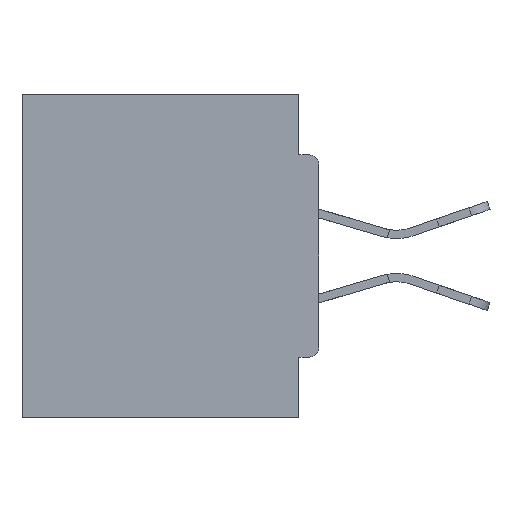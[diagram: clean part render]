
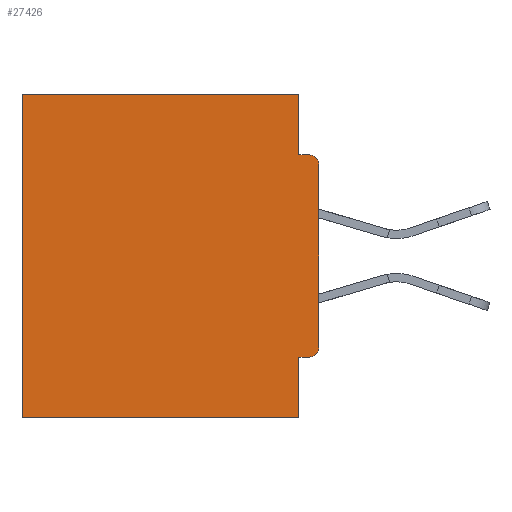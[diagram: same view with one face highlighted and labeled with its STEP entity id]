
A CAD part, left-side view. The second image highlights one B-rep face of the part: STEP entity #27426.
In plain terms, the highlighted planar face has unit normal (-1, 0, 0).
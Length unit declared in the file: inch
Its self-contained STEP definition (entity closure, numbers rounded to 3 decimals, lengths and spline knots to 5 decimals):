
#908 = DIRECTION ( 'NONE',  ( 0., -1., 0. ) ) ;
#1036 = EDGE_CURVE ( 'NONE', #26128, #29385, #31450, .T. ) ;
#2875 = VERTEX_POINT ( 'NONE', #4500 ) ;
#3977 = CARTESIAN_POINT ( 'NONE',  ( 0.298, 0., -0.0935 ) ) ;
#4500 = CARTESIAN_POINT ( 'NONE',  ( 0.298, 0.031, 0. ) ) ;
#4774 = LINE ( 'NONE', #9649, #39396 ) ;
#5343 = EDGE_CURVE ( 'NONE', #30835, #35171, #8415, .T. ) ;
#6039 = AXIS2_PLACEMENT_3D ( 'NONE', #40846, #12125, #31103 ) ;
#6791 = CARTESIAN_POINT ( 'NONE',  ( 0.298, 0.015, -0.3915 ) ) ;
#7238 = CARTESIAN_POINT ( 'NONE',  ( 0.298, 0.015, -0.0935 ) ) ;
#7319 = CARTESIAN_POINT ( 'NONE',  ( 0.298, 0.46, 0. ) ) ;
#7606 = ORIENTED_EDGE ( 'NONE', *, *, #35870, .T. ) ;
#7838 = DIRECTION ( 'NONE',  ( 0., 0., -1. ) ) ;
#8415 = LINE ( 'NONE', #36304, #37063 ) ;
#9649 = CARTESIAN_POINT ( 'NONE',  ( 0.298, 0.031, -0.5 ) ) ;
#10149 = CARTESIAN_POINT ( 'NONE',  ( 0.298, 0.015, -0.1085 ) ) ;
#10353 = DIRECTION ( 'NONE',  ( 0., 0., -1. ) ) ;
#11245 = ORIENTED_EDGE ( 'NONE', *, *, #20241, .T. ) ;
#11386 = ORIENTED_EDGE ( 'NONE', *, *, #24645, .F. ) ;
#12125 = DIRECTION ( 'NONE',  ( 1., 0., 0. ) ) ;
#12894 = EDGE_CURVE ( 'NONE', #2875, #20817, #28044, .T. ) ;
#13307 = ORIENTED_EDGE ( 'NONE', *, *, #5343, .F. ) ;
#14392 = CARTESIAN_POINT ( 'NONE',  ( 0.298, 0., 0. ) ) ;
#14441 = CARTESIAN_POINT ( 'NONE',  ( 0.298, 0.46, 0. ) ) ;
#14449 = VECTOR ( 'NONE', #39808, 39.37008 ) ;
#14754 = ORIENTED_EDGE ( 'NONE', *, *, #37496, .F. ) ;
#14957 = VERTEX_POINT ( 'NONE', #29770 ) ;
#15213 = EDGE_LOOP ( 'NONE', ( #7606, #28467, #11386, #28858, #11245, #13307, #23914, #29874, #31827, #14754 ) ) ;
#16209 = DIRECTION ( 'NONE',  ( -1., 0., 0. ) ) ;
#16326 = CARTESIAN_POINT ( 'NONE',  ( 0.298, 0.031, -0.5 ) ) ;
#20241 = EDGE_CURVE ( 'NONE', #20817, #35171, #28998, .T. ) ;
#20654 = DIRECTION ( 'NONE',  ( 0., 0., -1. ) ) ;
#20817 = VERTEX_POINT ( 'NONE', #7319 ) ;
#21018 = CARTESIAN_POINT ( 'NONE',  ( 0.298, 0., 0. ) ) ;
#21055 = VECTOR ( 'NONE', #908, 39.37008 ) ;
#21296 = DIRECTION ( 'NONE',  ( 0., 1., 0. ) ) ;
#22130 = AXIS2_PLACEMENT_3D ( 'NONE', #6791, #22304, #38011 ) ;
#22304 = DIRECTION ( 'NONE',  ( -1., 0., 0. ) ) ;
#22726 = CIRCLE ( 'NONE', #31453, 0.015 ) ;
#23914 = ORIENTED_EDGE ( 'NONE', *, *, #25435, .F. ) ;
#23992 = CARTESIAN_POINT ( 'NONE',  ( 0.298, 0.46, -0.5 ) ) ;
#24191 = CARTESIAN_POINT ( 'NONE',  ( 0.298, 0.031, -0.0935 ) ) ;
#24201 = VECTOR ( 'NONE', #10353, 39.37008 ) ;
#24645 = EDGE_CURVE ( 'NONE', #2875, #26128, #33553, .T. ) ;
#25435 = EDGE_CURVE ( 'NONE', #28665, #30835, #4774, .T. ) ;
#26027 = FACE_OUTER_BOUND ( 'NONE', #15213, .T. ) ;
#26128 = VERTEX_POINT ( 'NONE', #24191 ) ;
#27426 = ADVANCED_FACE ( 'NONE', ( #26027 ), #34250, .F. ) ;
#28044 = LINE ( 'NONE', #21018, #35411 ) ;
#28341 = LINE ( 'NONE', #30626, #14449 ) ;
#28467 = ORIENTED_EDGE ( 'NONE', *, *, #1036, .F. ) ;
#28665 = VERTEX_POINT ( 'NONE', #29125 ) ;
#28858 = ORIENTED_EDGE ( 'NONE', *, *, #12894, .T. ) ;
#28923 = DIRECTION ( 'NONE',  ( 0., 0., -1. ) ) ;
#28998 = LINE ( 'NONE', #14441, #36326 ) ;
#29125 = CARTESIAN_POINT ( 'NONE',  ( 0.298, 0.031, -0.4065 ) ) ;
#29385 = VERTEX_POINT ( 'NONE', #7238 ) ;
#29770 = CARTESIAN_POINT ( 'NONE',  ( 0.298, 0., -0.3915 ) ) ;
#29874 = ORIENTED_EDGE ( 'NONE', *, *, #38999, .F. ) ;
#30626 = CARTESIAN_POINT ( 'NONE',  ( 0.298, 0., -0.4065 ) ) ;
#30759 = CARTESIAN_POINT ( 'NONE',  ( 0.298, 0., -0.1085 ) ) ;
#30835 = VERTEX_POINT ( 'NONE', #16326 ) ;
#30977 = VECTOR ( 'NONE', #20654, 39.37008 ) ;
#31103 = DIRECTION ( 'NONE',  ( 0., 0., -1. ) ) ;
#31450 = LINE ( 'NONE', #3977, #21055 ) ;
#31453 = AXIS2_PLACEMENT_3D ( 'NONE', #10149, #16209, #35459 ) ;
#31827 = ORIENTED_EDGE ( 'NONE', *, *, #32901, .T. ) ;
#32092 = VERTEX_POINT ( 'NONE', #38429 ) ;
#32901 = EDGE_CURVE ( 'NONE', #32092, #14957, #36401, .T. ) ;
#32926 = LINE ( 'NONE', #14392, #30977 ) ;
#33553 = LINE ( 'NONE', #35662, #24201 ) ;
#34250 = PLANE ( 'NONE',  #6039 ) ;
#34569 = VERTEX_POINT ( 'NONE', #30759 ) ;
#35171 = VERTEX_POINT ( 'NONE', #23992 ) ;
#35411 = VECTOR ( 'NONE', #21296, 39.37008 ) ;
#35459 = DIRECTION ( 'NONE',  ( 0., 0., -1. ) ) ;
#35662 = CARTESIAN_POINT ( 'NONE',  ( 0.298, 0.031, -0.5 ) ) ;
#35870 = EDGE_CURVE ( 'NONE', #34569, #29385, #22726, .T. ) ;
#36180 = DIRECTION ( 'NONE',  ( 0., 1., 0. ) ) ;
#36304 = CARTESIAN_POINT ( 'NONE',  ( 0.298, 0., -0.5 ) ) ;
#36326 = VECTOR ( 'NONE', #7838, 39.37008 ) ;
#36401 = CIRCLE ( 'NONE', #22130, 0.015 ) ;
#37063 = VECTOR ( 'NONE', #36180, 39.37008 ) ;
#37496 = EDGE_CURVE ( 'NONE', #34569, #14957, #32926, .T. ) ;
#38011 = DIRECTION ( 'NONE',  ( 0., 0., -1. ) ) ;
#38429 = CARTESIAN_POINT ( 'NONE',  ( 0.298, 0.015, -0.4065 ) ) ;
#38999 = EDGE_CURVE ( 'NONE', #32092, #28665, #28341, .T. ) ;
#39396 = VECTOR ( 'NONE', #28923, 39.37008 ) ;
#39808 = DIRECTION ( 'NONE',  ( 0., 1., 0. ) ) ;
#40846 = CARTESIAN_POINT ( 'NONE',  ( 0.298, 0., 0. ) ) ;
